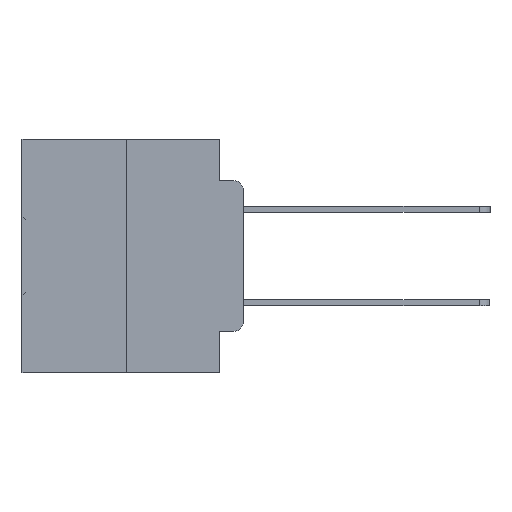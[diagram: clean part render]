
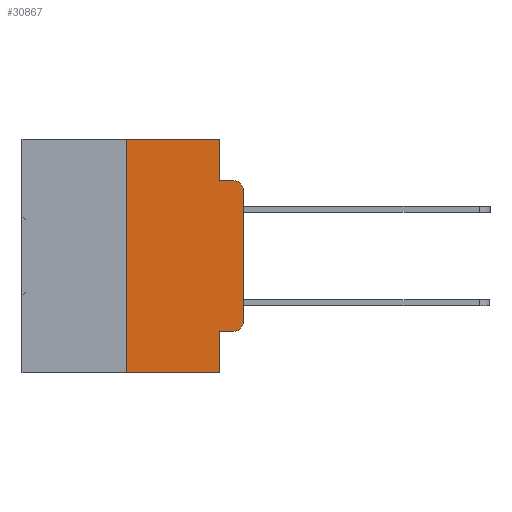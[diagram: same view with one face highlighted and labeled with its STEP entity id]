
A CAD part, left-side view. The second image highlights one B-rep face of the part: STEP entity #30867.
In plain terms, the highlighted planar face has unit normal (-1, 0, 0).
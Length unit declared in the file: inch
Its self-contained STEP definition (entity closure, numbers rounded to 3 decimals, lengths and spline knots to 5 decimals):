
#442 = DIRECTION ( 'NONE',  ( 0., -1., 0. ) ) ;
#755 = CIRCLE ( 'NONE', #13145, 0.02 ) ;
#1153 = VERTEX_POINT ( 'NONE', #14180 ) ;
#1303 = DIRECTION ( 'NONE',  ( -1., 0., 0. ) ) ;
#1852 = LINE ( 'NONE', #6840, #29831 ) ;
#2060 = PLANE ( 'NONE',  #17368 ) ;
#2498 = EDGE_CURVE ( 'NONE', #5340, #32201, #27390, .T. ) ;
#2603 = LINE ( 'NONE', #5588, #30574 ) ;
#2612 = CARTESIAN_POINT ( 'NONE',  ( 0., 0., -0.1085 ) ) ;
#2734 = ORIENTED_EDGE ( 'NONE', *, *, #7377, .F. ) ;
#2956 = CARTESIAN_POINT ( 'NONE',  ( 0., 0., -0.3915 ) ) ;
#3377 = ORIENTED_EDGE ( 'NONE', *, *, #19124, .T. ) ;
#3497 = LINE ( 'NONE', #13113, #23561 ) ;
#4263 = VECTOR ( 'NONE', #15509, 39.37008 ) ;
#4561 = CARTESIAN_POINT ( 'NONE',  ( 0., 0.25, 0. ) ) ;
#4829 = DIRECTION ( 'NONE',  ( 1., 0., 0. ) ) ;
#5050 = EDGE_CURVE ( 'NONE', #34071, #13184, #755, .T. ) ;
#5247 = VERTEX_POINT ( 'NONE', #2612 ) ;
#5340 = VERTEX_POINT ( 'NONE', #30197 ) ;
#5588 = CARTESIAN_POINT ( 'NONE',  ( 0., 0.473, 0. ) ) ;
#5612 = VERTEX_POINT ( 'NONE', #28482 ) ;
#6038 = VECTOR ( 'NONE', #442, 39.37008 ) ;
#6199 = VECTOR ( 'NONE', #27563, 39.37008 ) ;
#6840 = CARTESIAN_POINT ( 'NONE',  ( 0., 0., 0. ) ) ;
#7064 = VERTEX_POINT ( 'NONE', #4561 ) ;
#7377 = EDGE_CURVE ( 'NONE', #1153, #26580, #27813, .T. ) ;
#8578 = ORIENTED_EDGE ( 'NONE', *, *, #25580, .F. ) ;
#8711 = ORIENTED_EDGE ( 'NONE', *, *, #24238, .T. ) ;
#9639 = CARTESIAN_POINT ( 'NONE',  ( 0., 0.051, -0.0885 ) ) ;
#9676 = CARTESIAN_POINT ( 'NONE',  ( 0., 0.051, -0.5 ) ) ;
#10213 = EDGE_LOOP ( 'NONE', ( #8711, #23279, #13466, #2734, #8578, #28885, #3377, #19480, #10812, #11744 ) ) ;
#10812 = ORIENTED_EDGE ( 'NONE', *, *, #25106, .T. ) ;
#11470 = EDGE_CURVE ( 'NONE', #5247, #5612, #24860, .T. ) ;
#11744 = ORIENTED_EDGE ( 'NONE', *, *, #5050, .T. ) ;
#12202 = DIRECTION ( 'NONE',  ( -1., 0., 0. ) ) ;
#13113 = CARTESIAN_POINT ( 'NONE',  ( 0., 0.051, -0.4115 ) ) ;
#13145 = AXIS2_PLACEMENT_3D ( 'NONE', #17672, #1303, #20438 ) ;
#13184 = VERTEX_POINT ( 'NONE', #2956 ) ;
#13466 = ORIENTED_EDGE ( 'NONE', *, *, #23099, .F. ) ;
#13539 = EDGE_CURVE ( 'NONE', #32402, #7064, #18803, .T. ) ;
#14094 = CARTESIAN_POINT ( 'NONE',  ( 0., 0.473, -0.5 ) ) ;
#14180 = CARTESIAN_POINT ( 'NONE',  ( 0., 0.051, 0. ) ) ;
#15072 = DIRECTION ( 'NONE',  ( 0., 0., 1. ) ) ;
#15255 = CARTESIAN_POINT ( 'NONE',  ( 0., 0.051, 0. ) ) ;
#15509 = DIRECTION ( 'NONE',  ( 0., 0., 1. ) ) ;
#17368 = AXIS2_PLACEMENT_3D ( 'NONE', #21183, #4829, #23880 ) ;
#17672 = CARTESIAN_POINT ( 'NONE',  ( 0., 0.02, -0.3915 ) ) ;
#18803 = LINE ( 'NONE', #20871, #4263 ) ;
#19124 = EDGE_CURVE ( 'NONE', #32402, #32201, #28490, .T. ) ;
#19376 = VECTOR ( 'NONE', #26142, 39.37008 ) ;
#19480 = ORIENTED_EDGE ( 'NONE', *, *, #2498, .F. ) ;
#20438 = DIRECTION ( 'NONE',  ( 0., 0., -1. ) ) ;
#20871 = CARTESIAN_POINT ( 'NONE',  ( 0., 0.25, 0. ) ) ;
#21183 = CARTESIAN_POINT ( 'NONE',  ( 0., 0.473, 0. ) ) ;
#23099 = EDGE_CURVE ( 'NONE', #26580, #5612, #26663, .T. ) ;
#23208 = DIRECTION ( 'NONE',  ( 0., -1., 0. ) ) ;
#23279 = ORIENTED_EDGE ( 'NONE', *, *, #11470, .T. ) ;
#23373 = CARTESIAN_POINT ( 'NONE',  ( 0., 0.02, -0.4115 ) ) ;
#23561 = VECTOR ( 'NONE', #34584, 39.37008 ) ;
#23853 = CARTESIAN_POINT ( 'NONE',  ( 0., 0.051, -0.0885 ) ) ;
#23880 = DIRECTION ( 'NONE',  ( 0., 0., -1. ) ) ;
#24179 = CARTESIAN_POINT ( 'NONE',  ( 0., 0.25, -0.5 ) ) ;
#24238 = EDGE_CURVE ( 'NONE', #13184, #5247, #1852, .T. ) ;
#24860 = CIRCLE ( 'NONE', #26228, 0.02 ) ;
#25106 = EDGE_CURVE ( 'NONE', #5340, #34071, #3497, .T. ) ;
#25580 = EDGE_CURVE ( 'NONE', #7064, #1153, #2603, .T. ) ;
#25822 = VECTOR ( 'NONE', #23208, 39.37008 ) ;
#26142 = DIRECTION ( 'NONE',  ( 0., 0., -1. ) ) ;
#26228 = AXIS2_PLACEMENT_3D ( 'NONE', #28384, #12202, #31007 ) ;
#26580 = VERTEX_POINT ( 'NONE', #23853 ) ;
#26663 = LINE ( 'NONE', #9639, #25822 ) ;
#27390 = LINE ( 'NONE', #15255, #19376 ) ;
#27563 = DIRECTION ( 'NONE',  ( 0., 0., -1. ) ) ;
#27813 = LINE ( 'NONE', #30183, #6199 ) ;
#28384 = CARTESIAN_POINT ( 'NONE',  ( 0., 0.02, -0.1085 ) ) ;
#28482 = CARTESIAN_POINT ( 'NONE',  ( 0., 0.02, -0.0885 ) ) ;
#28490 = LINE ( 'NONE', #14094, #6038 ) ;
#28885 = ORIENTED_EDGE ( 'NONE', *, *, #13539, .F. ) ;
#29126 = FACE_OUTER_BOUND ( 'NONE', #10213, .T. ) ;
#29831 = VECTOR ( 'NONE', #15072, 39.37008 ) ;
#30183 = CARTESIAN_POINT ( 'NONE',  ( 0., 0.051, 0. ) ) ;
#30197 = CARTESIAN_POINT ( 'NONE',  ( 0., 0.051, -0.4115 ) ) ;
#30574 = VECTOR ( 'NONE', #32594, 39.37008 ) ;
#30867 = ADVANCED_FACE ( 'NONE', ( #29126 ), #2060, .F. ) ;
#31007 = DIRECTION ( 'NONE',  ( 0., 0., -1. ) ) ;
#32201 = VERTEX_POINT ( 'NONE', #9676 ) ;
#32402 = VERTEX_POINT ( 'NONE', #24179 ) ;
#32594 = DIRECTION ( 'NONE',  ( 0., -1., 0. ) ) ;
#34071 = VERTEX_POINT ( 'NONE', #23373 ) ;
#34584 = DIRECTION ( 'NONE',  ( 0., -1., 0. ) ) ;
